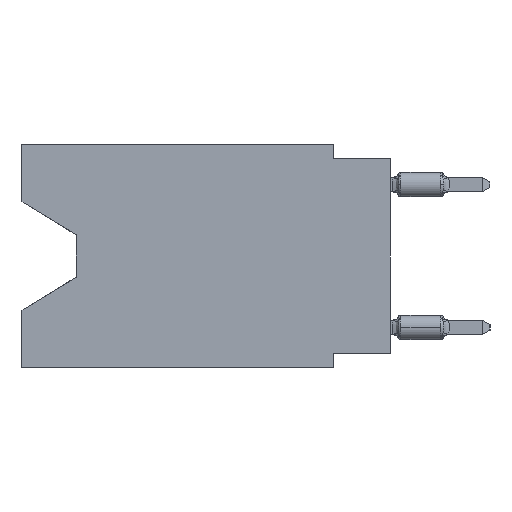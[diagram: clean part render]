
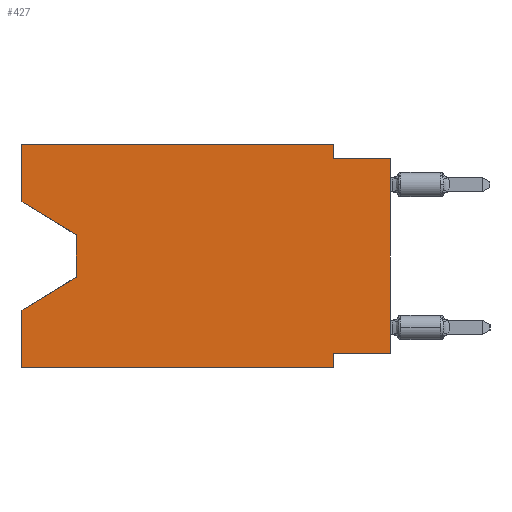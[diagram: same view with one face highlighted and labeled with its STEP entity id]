
A CAD part, left-side view. The second image highlights one B-rep face of the part: STEP entity #427.
In plain terms, the highlighted planar face has unit normal (-1, 0, 0).
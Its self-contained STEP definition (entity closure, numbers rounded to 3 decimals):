
#51 = CARTESIAN_POINT ( 'NONE',  ( 0., 16.383, 0. ) ) ;
#173 = DIRECTION ( 'NONE',  ( 0., 0., -1. ) ) ;
#204 = VECTOR ( 'NONE', #8868, 1000. ) ;
#427 = ADVANCED_FACE ( 'NONE', ( #14603 ), #1661, .F. ) ;
#558 = LINE ( 'NONE', #17528, #1979 ) ;
#786 = DIRECTION ( 'NONE',  ( 0., 0., 1. ) ) ;
#866 = EDGE_CURVE ( 'NONE', #7803, #23202, #2204, .T. ) ;
#954 = ORIENTED_EDGE ( 'NONE', *, *, #866, .F. ) ;
#1080 = DIRECTION ( 'NONE',  ( 0., 0., -1. ) ) ;
#1171 = CARTESIAN_POINT ( 'NONE',  ( 0., 0., -0.635 ) ) ;
#1201 = LINE ( 'NONE', #12289, #5774 ) ;
#1661 = PLANE ( 'NONE',  #23417 ) ;
#1894 = DIRECTION ( 'NONE',  ( 0., 1., 0. ) ) ;
#1979 = VECTOR ( 'NONE', #786, 1000. ) ;
#2125 = CARTESIAN_POINT ( 'NONE',  ( 0., 2.54, -0.635 ) ) ;
#2204 = LINE ( 'NONE', #17101, #21860 ) ;
#2465 = LINE ( 'NONE', #21285, #6836 ) ;
#2529 = EDGE_CURVE ( 'NONE', #14315, #23633, #8488, .T. ) ;
#3123 = EDGE_CURVE ( 'NONE', #19350, #23202, #4685, .T. ) ;
#3434 = ORIENTED_EDGE ( 'NONE', *, *, #3123, .T. ) ;
#4384 = ORIENTED_EDGE ( 'NONE', *, *, #2529, .F. ) ;
#4645 = ORIENTED_EDGE ( 'NONE', *, *, #17763, .F. ) ;
#4685 = LINE ( 'NONE', #6738, #22737 ) ;
#4709 = CARTESIAN_POINT ( 'NONE',  ( 0., 16.383, -9.906 ) ) ;
#5774 = VECTOR ( 'NONE', #1080, 1000. ) ;
#5894 = EDGE_CURVE ( 'NONE', #21924, #21861, #20838, .T. ) ;
#6738 = CARTESIAN_POINT ( 'NONE',  ( 0., 13.97, -5.893 ) ) ;
#6836 = VECTOR ( 'NONE', #17481, 1000. ) ;
#6877 = VECTOR ( 'NONE', #23833, 1000. ) ;
#7716 = ORIENTED_EDGE ( 'NONE', *, *, #7751, .T. ) ;
#7751 = EDGE_CURVE ( 'NONE', #21924, #21858, #558, .T. ) ;
#7754 = ORIENTED_EDGE ( 'NONE', *, *, #5894, .F. ) ;
#7803 = VERTEX_POINT ( 'NONE', #4709 ) ;
#8250 = CARTESIAN_POINT ( 'NONE',  ( 0., 2.54, 0. ) ) ;
#8473 = CARTESIAN_POINT ( 'NONE',  ( 0., 16.383, -9.906 ) ) ;
#8488 = LINE ( 'NONE', #8250, #16439 ) ;
#8598 = CARTESIAN_POINT ( 'NONE',  ( 0., 2.54, -9.271 ) ) ;
#8868 = DIRECTION ( 'NONE',  ( 0., -1., 0. ) ) ;
#9128 = VERTEX_POINT ( 'NONE', #23667 ) ;
#9222 = ORIENTED_EDGE ( 'NONE', *, *, #20396, .T. ) ;
#9451 = CARTESIAN_POINT ( 'NONE',  ( 0., 0., -9.271 ) ) ;
#10149 = CARTESIAN_POINT ( 'NONE',  ( 0., 16.383, -2.546 ) ) ;
#10812 = LINE ( 'NONE', #20014, #204 ) ;
#11058 = VECTOR ( 'NONE', #21689, 1000. ) ;
#11062 = LINE ( 'NONE', #22229, #6877 ) ;
#11573 = LINE ( 'NONE', #17091, #15800 ) ;
#11778 = CARTESIAN_POINT ( 'NONE',  ( 0., 16.383, -7.36 ) ) ;
#12181 = EDGE_CURVE ( 'NONE', #23633, #21858, #11573, .T. ) ;
#12289 = CARTESIAN_POINT ( 'NONE',  ( 0., 2.54, -9.906 ) ) ;
#12614 = VERTEX_POINT ( 'NONE', #20994 ) ;
#12664 = ORIENTED_EDGE ( 'NONE', *, *, #18289, .F. ) ;
#12769 = CARTESIAN_POINT ( 'NONE',  ( 0., 0., -9.271 ) ) ;
#12792 = EDGE_CURVE ( 'NONE', #7803, #12614, #23919, .T. ) ;
#13133 = ORIENTED_EDGE ( 'NONE', *, *, #21284, .F. ) ;
#13255 = DIRECTION ( 'NONE',  ( 1., 0., 0. ) ) ;
#14209 = EDGE_LOOP ( 'NONE', ( #9222, #21706, #3434, #954, #17880, #13133, #7754, #7716, #23789, #4384, #4645, #12664 ) ) ;
#14315 = VERTEX_POINT ( 'NONE', #23646 ) ;
#14603 = FACE_OUTER_BOUND ( 'NONE', #14209, .T. ) ;
#14924 = CARTESIAN_POINT ( 'NONE',  ( 0., 13.97, -5.893 ) ) ;
#15792 = LINE ( 'NONE', #10149, #19403 ) ;
#15800 = VECTOR ( 'NONE', #19065, 1000. ) ;
#16334 = VECTOR ( 'NONE', #1894, 1000. ) ;
#16439 = VECTOR ( 'NONE', #21241, 1000. ) ;
#16942 = DIRECTION ( 'NONE',  ( 0., -0.855, -0.519 ) ) ;
#17091 = CARTESIAN_POINT ( 'NONE',  ( 0., 0., -0.635 ) ) ;
#17101 = CARTESIAN_POINT ( 'NONE',  ( 0., 16.383, 0. ) ) ;
#17481 = DIRECTION ( 'NONE',  ( 0., 0., 1. ) ) ;
#17528 = CARTESIAN_POINT ( 'NONE',  ( 0., 0., 0. ) ) ;
#17634 = CARTESIAN_POINT ( 'NONE',  ( 0., 16.383, 0. ) ) ;
#17763 = EDGE_CURVE ( 'NONE', #22176, #14315, #10812, .T. ) ;
#17880 = ORIENTED_EDGE ( 'NONE', *, *, #12792, .T. ) ;
#18289 = EDGE_CURVE ( 'NONE', #9128, #22176, #2465, .T. ) ;
#19065 = DIRECTION ( 'NONE',  ( 0., -1., 0. ) ) ;
#19078 = DIRECTION ( 'NONE',  ( 0., 0., 1. ) ) ;
#19350 = VERTEX_POINT ( 'NONE', #14924 ) ;
#19403 = VECTOR ( 'NONE', #16942, 1000. ) ;
#19602 = DIRECTION ( 'NONE',  ( 0., 0.855, -0.519 ) ) ;
#19617 = VERTEX_POINT ( 'NONE', #23254 ) ;
#20014 = CARTESIAN_POINT ( 'NONE',  ( 0., 16.383, 0. ) ) ;
#20195 = EDGE_CURVE ( 'NONE', #19617, #19350, #11062, .T. ) ;
#20396 = EDGE_CURVE ( 'NONE', #9128, #19617, #15792, .T. ) ;
#20838 = LINE ( 'NONE', #9451, #16334 ) ;
#20994 = CARTESIAN_POINT ( 'NONE',  ( 0., 2.54, -9.906 ) ) ;
#21241 = DIRECTION ( 'NONE',  ( 0., 0., -1. ) ) ;
#21284 = EDGE_CURVE ( 'NONE', #21861, #12614, #1201, .T. ) ;
#21285 = CARTESIAN_POINT ( 'NONE',  ( 0., 16.383, 0. ) ) ;
#21689 = DIRECTION ( 'NONE',  ( 0., -1., 0. ) ) ;
#21706 = ORIENTED_EDGE ( 'NONE', *, *, #20195, .T. ) ;
#21858 = VERTEX_POINT ( 'NONE', #1171 ) ;
#21860 = VECTOR ( 'NONE', #19078, 1000. ) ;
#21861 = VERTEX_POINT ( 'NONE', #8598 ) ;
#21924 = VERTEX_POINT ( 'NONE', #12769 ) ;
#22176 = VERTEX_POINT ( 'NONE', #17634 ) ;
#22229 = CARTESIAN_POINT ( 'NONE',  ( 0., 13.97, -4.013 ) ) ;
#22737 = VECTOR ( 'NONE', #19602, 1000. ) ;
#23202 = VERTEX_POINT ( 'NONE', #11778 ) ;
#23254 = CARTESIAN_POINT ( 'NONE',  ( 0., 13.97, -4.013 ) ) ;
#23417 = AXIS2_PLACEMENT_3D ( 'NONE', #51, #13255, #173 ) ;
#23633 = VERTEX_POINT ( 'NONE', #2125 ) ;
#23646 = CARTESIAN_POINT ( 'NONE',  ( 0., 2.54, 0. ) ) ;
#23667 = CARTESIAN_POINT ( 'NONE',  ( 0., 16.383, -2.546 ) ) ;
#23789 = ORIENTED_EDGE ( 'NONE', *, *, #12181, .F. ) ;
#23833 = DIRECTION ( 'NONE',  ( 0., 0., -1. ) ) ;
#23919 = LINE ( 'NONE', #8473, #11058 ) ;
